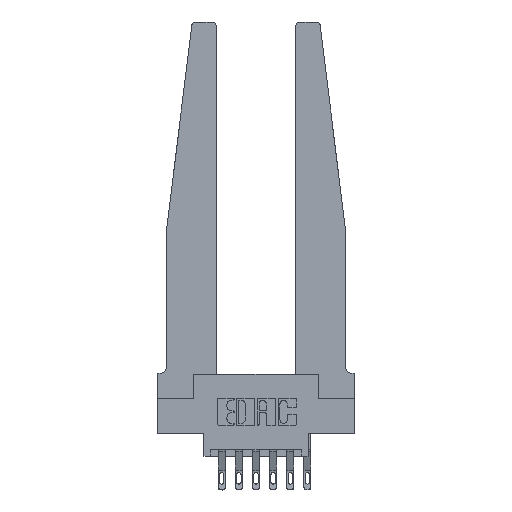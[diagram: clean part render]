
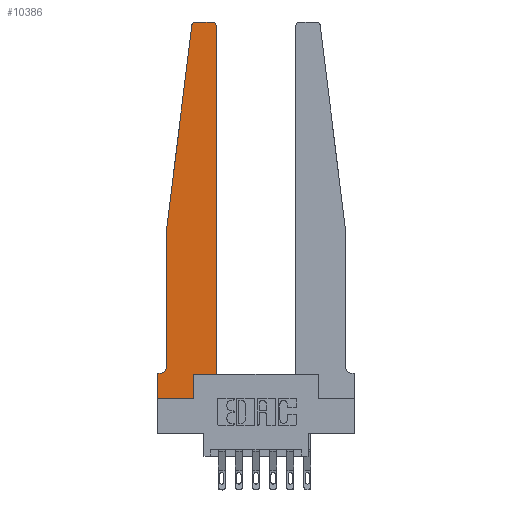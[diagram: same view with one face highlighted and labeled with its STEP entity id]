
A CAD part, top view. The second image highlights one B-rep face of the part: STEP entity #10386.
In plain terms, the highlighted planar face has unit normal (0, 0, 1).
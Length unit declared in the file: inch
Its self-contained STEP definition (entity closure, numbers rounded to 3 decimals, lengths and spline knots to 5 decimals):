
#95 = CARTESIAN_POINT ( 'NONE',  ( 0.27653, 2.75, 0.37 ) ) ;
#341 = CARTESIAN_POINT ( 'NONE',  ( 0.425, 0.18, 0.37 ) ) ;
#560 = ORIENTED_EDGE ( 'NONE', *, *, #1796, .T. ) ;
#789 = AXIS2_PLACEMENT_3D ( 'NONE', #1150, #13877, #6409 ) ;
#925 = CARTESIAN_POINT ( 'NONE',  ( 0.425, 2.72, 0.37 ) ) ;
#946 = EDGE_CURVE ( 'NONE', #11158, #1540, #7692, .T. ) ;
#1068 = DIRECTION ( 'NONE',  ( 1., 0., 0. ) ) ;
#1070 = DIRECTION ( 'NONE',  ( 0., -1., 0. ) ) ;
#1097 = DIRECTION ( 'NONE',  ( 0., 0., 1. ) ) ;
#1127 = VERTEX_POINT ( 'NONE', #10666 ) ;
#1150 = CARTESIAN_POINT ( 'NONE',  ( 0.27653, 2.72, 0.37 ) ) ;
#1540 = VERTEX_POINT ( 'NONE', #12204 ) ;
#1785 = ORIENTED_EDGE ( 'NONE', *, *, #2031, .T. ) ;
#1796 = EDGE_CURVE ( 'NONE', #1127, #4466, #4208, .T. ) ;
#1807 = VERTEX_POINT ( 'NONE', #4344 ) ;
#1856 = CARTESIAN_POINT ( 'NONE',  ( 0.395, 2.75, 0.37 ) ) ;
#1928 = EDGE_LOOP ( 'NONE', ( #11566, #12841, #10324, #6041, #1785, #560, #2256, #7347, #12578, #11046, #13221, #3988 ) ) ;
#2031 = EDGE_CURVE ( 'NONE', #1540, #1127, #13318, .T. ) ;
#2075 = DIRECTION ( 'NONE',  ( 1., 0., 0. ) ) ;
#2100 = VECTOR ( 'NONE', #4626, 39.37008 ) ;
#2256 = ORIENTED_EDGE ( 'NONE', *, *, #7430, .T. ) ;
#2508 = DIRECTION ( 'NONE',  ( 1., 0., 0. ) ) ;
#2550 = AXIS2_PLACEMENT_3D ( 'NONE', #7490, #1097, #2075 ) ;
#2679 = LINE ( 'NONE', #10399, #11983 ) ;
#2710 = CARTESIAN_POINT ( 'NONE',  ( 0.015, 0.2375, 0.37 ) ) ;
#3162 = CARTESIAN_POINT ( 'NONE',  ( 0., 0., 0.37 ) ) ;
#3496 = CIRCLE ( 'NONE', #11611, 0.03 ) ;
#3521 = CARTESIAN_POINT ( 'NONE',  ( 0.395, 2.72, 0.37 ) ) ;
#3552 = LINE ( 'NONE', #7648, #12972 ) ;
#3818 = VECTOR ( 'NONE', #5406, 39.37008 ) ;
#3906 = EDGE_CURVE ( 'NONE', #9741, #1807, #2679, .T. ) ;
#3988 = ORIENTED_EDGE ( 'NONE', *, *, #12276, .T. ) ;
#4174 = DIRECTION ( 'NONE',  ( 1., 0., 0. ) ) ;
#4208 = LINE ( 'NONE', #6384, #3818 ) ;
#4305 = DIRECTION ( 'NONE',  ( 0., -1., 0. ) ) ;
#4344 = CARTESIAN_POINT ( 'NONE',  ( 0.2605, 0.18, 0.37 ) ) ;
#4466 = VERTEX_POINT ( 'NONE', #8184 ) ;
#4572 = DIRECTION ( 'NONE',  ( -1., 0., 0. ) ) ;
#4626 = DIRECTION ( 'NONE',  ( 0., 1., 0. ) ) ;
#4727 = EDGE_CURVE ( 'NONE', #9111, #6160, #5674, .T. ) ;
#5406 = DIRECTION ( 'NONE',  ( -1., 0., 0. ) ) ;
#5475 = VECTOR ( 'NONE', #4572, 39.37008 ) ;
#5674 = LINE ( 'NONE', #341, #2100 ) ;
#6041 = ORIENTED_EDGE ( 'NONE', *, *, #946, .T. ) ;
#6060 = DIRECTION ( 'NONE',  ( 0., 1., 0. ) ) ;
#6160 = VERTEX_POINT ( 'NONE', #925 ) ;
#6384 = CARTESIAN_POINT ( 'NONE',  ( 0.065, 0.1875, 0.37 ) ) ;
#6409 = DIRECTION ( 'NONE',  ( 1., 0., 0. ) ) ;
#6469 = LINE ( 'NONE', #8893, #5475 ) ;
#6537 = VECTOR ( 'NONE', #4305, 39.37008 ) ;
#6623 = CARTESIAN_POINT ( 'NONE',  ( 0.065, 1.25, 0.37 ) ) ;
#6869 = VERTEX_POINT ( 'NONE', #1856 ) ;
#7024 = EDGE_CURVE ( 'NONE', #9592, #8007, #9821, .T. ) ;
#7347 = ORIENTED_EDGE ( 'NONE', *, *, #8764, .T. ) ;
#7430 = EDGE_CURVE ( 'NONE', #4466, #11600, #10735, .T. ) ;
#7433 = CARTESIAN_POINT ( 'NONE',  ( 0.425, 0.18, 0.37 ) ) ;
#7490 = CARTESIAN_POINT ( 'NONE',  ( 0., 0.1875, 0.37 ) ) ;
#7648 = CARTESIAN_POINT ( 'NONE',  ( 0.065, 1.25, 0.37 ) ) ;
#7692 = LINE ( 'NONE', #6623, #6537 ) ;
#8007 = VERTEX_POINT ( 'NONE', #8919 ) ;
#8184 = CARTESIAN_POINT ( 'NONE',  ( 0., 0.1875, 0.37 ) ) ;
#8516 = LINE ( 'NONE', #11570, #12489 ) ;
#8548 = FACE_OUTER_BOUND ( 'NONE', #1928, .T. ) ;
#8764 = EDGE_CURVE ( 'NONE', #11600, #9741, #10934, .T. ) ;
#8778 = DIRECTION ( 'NONE',  ( -0.122, -0.992, 0. ) ) ;
#8893 = CARTESIAN_POINT ( 'NONE',  ( 0.25, 2.75, 0.37 ) ) ;
#8919 = CARTESIAN_POINT ( 'NONE',  ( 0.24675, 2.72367, 0.37 ) ) ;
#8969 = VECTOR ( 'NONE', #2508, 39.37008 ) ;
#9111 = VERTEX_POINT ( 'NONE', #7433 ) ;
#9327 = EDGE_CURVE ( 'NONE', #8007, #11158, #3552, .T. ) ;
#9366 = DIRECTION ( 'NONE',  ( 0., 0., -1. ) ) ;
#9592 = VERTEX_POINT ( 'NONE', #95 ) ;
#9741 = VERTEX_POINT ( 'NONE', #10187 ) ;
#9821 = CIRCLE ( 'NONE', #789, 0.03 ) ;
#10187 = CARTESIAN_POINT ( 'NONE',  ( 0.2605, 0., 0.37 ) ) ;
#10324 = ORIENTED_EDGE ( 'NONE', *, *, #9327, .T. ) ;
#10386 = ADVANCED_FACE ( 'NONE', ( #8548 ), #13808, .T. ) ;
#10399 = CARTESIAN_POINT ( 'NONE',  ( 0.2605, 0.18, 0.37 ) ) ;
#10666 = CARTESIAN_POINT ( 'NONE',  ( 0.015, 0.1875, 0.37 ) ) ;
#10735 = LINE ( 'NONE', #3162, #12058 ) ;
#10859 = CARTESIAN_POINT ( 'NONE',  ( 0., 0., 0.37 ) ) ;
#10934 = LINE ( 'NONE', #10859, #8969 ) ;
#11021 = EDGE_CURVE ( 'NONE', #6869, #9592, #6469, .T. ) ;
#11046 = ORIENTED_EDGE ( 'NONE', *, *, #12577, .T. ) ;
#11069 = CARTESIAN_POINT ( 'NONE',  ( 0., 0., 0.37 ) ) ;
#11158 = VERTEX_POINT ( 'NONE', #13346 ) ;
#11497 = AXIS2_PLACEMENT_3D ( 'NONE', #2710, #9366, #13604 ) ;
#11566 = ORIENTED_EDGE ( 'NONE', *, *, #11021, .T. ) ;
#11570 = CARTESIAN_POINT ( 'NONE',  ( 0.425, 0.18, 0.37 ) ) ;
#11600 = VERTEX_POINT ( 'NONE', #11069 ) ;
#11611 = AXIS2_PLACEMENT_3D ( 'NONE', #3521, #11997, #4174 ) ;
#11983 = VECTOR ( 'NONE', #6060, 39.37008 ) ;
#11997 = DIRECTION ( 'NONE',  ( 0., 0., 1. ) ) ;
#12058 = VECTOR ( 'NONE', #1070, 39.37008 ) ;
#12204 = CARTESIAN_POINT ( 'NONE',  ( 0.065, 0.2375, 0.37 ) ) ;
#12276 = EDGE_CURVE ( 'NONE', #6160, #6869, #3496, .T. ) ;
#12489 = VECTOR ( 'NONE', #1068, 39.37008 ) ;
#12577 = EDGE_CURVE ( 'NONE', #1807, #9111, #8516, .T. ) ;
#12578 = ORIENTED_EDGE ( 'NONE', *, *, #3906, .T. ) ;
#12841 = ORIENTED_EDGE ( 'NONE', *, *, #7024, .T. ) ;
#12972 = VECTOR ( 'NONE', #8778, 39.37008 ) ;
#13221 = ORIENTED_EDGE ( 'NONE', *, *, #4727, .T. ) ;
#13318 = CIRCLE ( 'NONE', #11497, 0.05 ) ;
#13346 = CARTESIAN_POINT ( 'NONE',  ( 0.065, 1.25, 0.37 ) ) ;
#13604 = DIRECTION ( 'NONE',  ( -1., 0., 0. ) ) ;
#13808 = PLANE ( 'NONE',  #2550 ) ;
#13877 = DIRECTION ( 'NONE',  ( 0., 0., 1. ) ) ;
